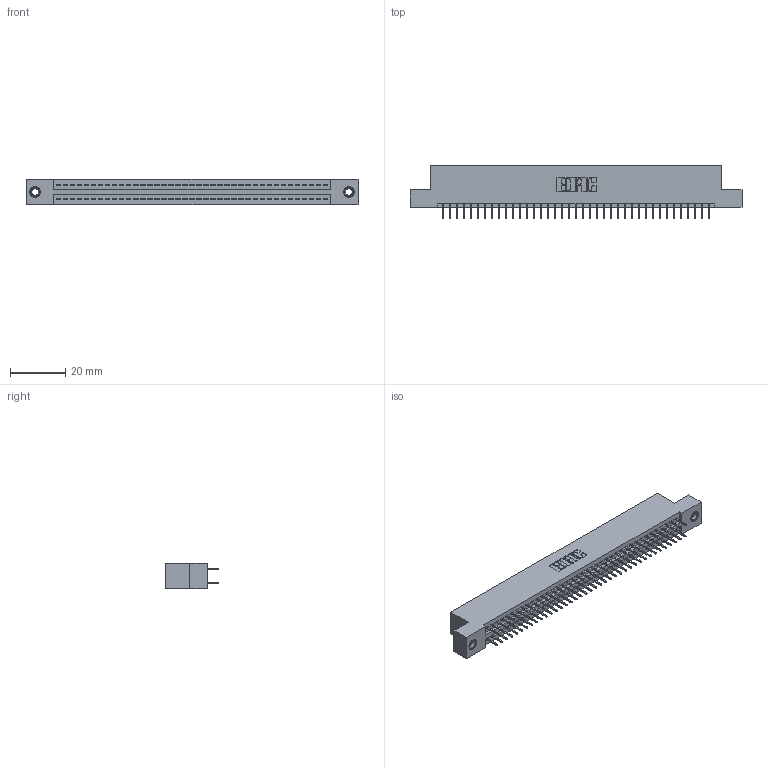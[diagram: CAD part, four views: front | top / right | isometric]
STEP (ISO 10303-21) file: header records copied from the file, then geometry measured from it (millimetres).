
FILE_DESCRIPTION (( 'STEP AP203' ), '1' );
FILE_NAME ('395-078-524-207.STEP', '2019-10-25T02:04:53', ( '' ), ( '' ), 'SwSTEP 2.0', 'SolidWorks 2016', '' );
FILE_SCHEMA (( 'CONFIG_CONTROL_DESIGN' ));
Length unit declared in the file: inch
Products named in the file (4): 345 Part_Flush Mounting Lugs - 0.156 Dia-TI; 345-292-001_345-293-124; 345-250-001_345-250-005-103; 395-078-524-207
Assembly tree (81 placements, depth 2):
  395-078-524-207
    345 Part_Flush Mounting Lugs - 0.156 Dia-TI
    345-292-001_345-293-124  x78
    345-250-001_345-250-005-103  x2
Bounding box: 120.27 x 19.35 x 9.4 mm (x, y, z)
Volume: 11523.7 mm3; surface area: 16692.1 mm2
Topology: 81 solids, 81 shells, 4398 faces, 12411 edges, 7954 vertices
Faces by surface type: plane 3154, cylinder 1228, cone 12, torus 4
Entity records: 32264 total; most frequent: CARTESIAN_POINT 5391, ORIENTED_EDGE 5318, DIRECTION 4785, EDGE_CURVE 2659, LINE 2355, VECTOR 2355, VERTEX_POINT 1764, AXIS2_PLACEMENT_3D 1215
